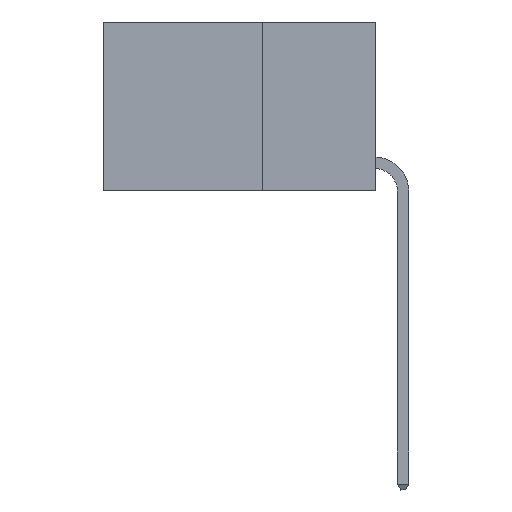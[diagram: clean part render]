
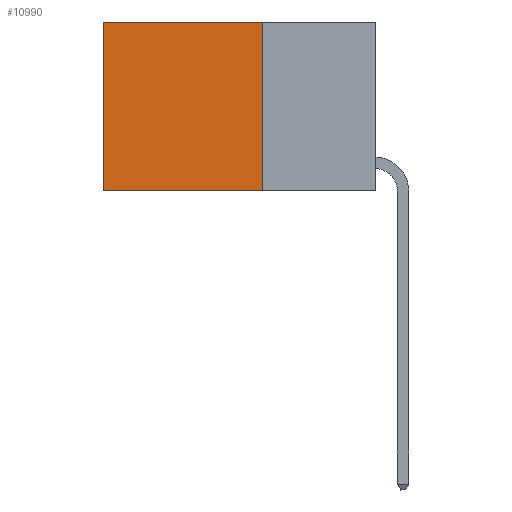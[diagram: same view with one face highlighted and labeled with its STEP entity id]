
A CAD part, left-side view. The second image highlights one B-rep face of the part: STEP entity #10990.
In plain terms, the highlighted planar face has unit normal (-1, 0, 0).
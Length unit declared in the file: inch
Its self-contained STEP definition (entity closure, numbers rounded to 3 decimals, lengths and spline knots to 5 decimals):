
#41 = LINE ( 'NONE', #14664, #10554 ) ;
#1117 = AXIS2_PLACEMENT_3D ( 'NONE', #23988, #11223, #20136 ) ;
#3269 = LINE ( 'NONE', #23696, #13465 ) ;
#3692 = VERTEX_POINT ( 'NONE', #24708 ) ;
#4666 = VERTEX_POINT ( 'NONE', #6920 ) ;
#5207 = VERTEX_POINT ( 'NONE', #9604 ) ;
#6920 = CARTESIAN_POINT ( 'NONE',  ( 0.2625, 0.25, -0.37 ) ) ;
#7227 = EDGE_CURVE ( 'NONE', #16724, #4666, #41, .T. ) ;
#7778 = VECTOR ( 'NONE', #10837, 39.37008 ) ;
#9604 = CARTESIAN_POINT ( 'NONE',  ( 0.2625, 0.6, 0. ) ) ;
#9693 = ORIENTED_EDGE ( 'NONE', *, *, #7227, .F. ) ;
#10187 = LINE ( 'NONE', #18152, #18713 ) ;
#10554 = VECTOR ( 'NONE', #22639, 39.37008 ) ;
#10837 = DIRECTION ( 'NONE',  ( 0., 0., -1. ) ) ;
#10990 = ADVANCED_FACE ( 'NONE', ( #24119 ), #21651, .F. ) ;
#11223 = DIRECTION ( 'NONE',  ( 1., 0., 0. ) ) ;
#11754 = ORIENTED_EDGE ( 'NONE', *, *, #15854, .F. ) ;
#12767 = CARTESIAN_POINT ( 'NONE',  ( 0.2625, 0.6, 0. ) ) ;
#12965 = ORIENTED_EDGE ( 'NONE', *, *, #16466, .T. ) ;
#13465 = VECTOR ( 'NONE', #19577, 39.37008 ) ;
#14553 = LINE ( 'NONE', #12767, #7778 ) ;
#14664 = CARTESIAN_POINT ( 'NONE',  ( 0.2625, 0.25, 0. ) ) ;
#15854 = EDGE_CURVE ( 'NONE', #4666, #3692, #10187, .T. ) ;
#16055 = EDGE_CURVE ( 'NONE', #16724, #5207, #3269, .T. ) ;
#16466 = EDGE_CURVE ( 'NONE', #5207, #3692, #14553, .T. ) ;
#16724 = VERTEX_POINT ( 'NONE', #20158 ) ;
#18152 = CARTESIAN_POINT ( 'NONE',  ( 0.2625, 0.25, -0.37 ) ) ;
#18432 = DIRECTION ( 'NONE',  ( 0., 1., 0. ) ) ;
#18713 = VECTOR ( 'NONE', #18432, 39.37008 ) ;
#19577 = DIRECTION ( 'NONE',  ( 0., 1., 0. ) ) ;
#19862 = ORIENTED_EDGE ( 'NONE', *, *, #16055, .T. ) ;
#19988 = EDGE_LOOP ( 'NONE', ( #12965, #11754, #9693, #19862 ) ) ;
#20136 = DIRECTION ( 'NONE',  ( 0., 0., -1. ) ) ;
#20158 = CARTESIAN_POINT ( 'NONE',  ( 0.2625, 0.25, 0. ) ) ;
#21651 = PLANE ( 'NONE',  #1117 ) ;
#22639 = DIRECTION ( 'NONE',  ( 0., 0., -1. ) ) ;
#23696 = CARTESIAN_POINT ( 'NONE',  ( 0.2625, 0.25, 0. ) ) ;
#23988 = CARTESIAN_POINT ( 'NONE',  ( 0.2625, 0.25, 0. ) ) ;
#24119 = FACE_OUTER_BOUND ( 'NONE', #19988, .T. ) ;
#24708 = CARTESIAN_POINT ( 'NONE',  ( 0.2625, 0.6, -0.37 ) ) ;
